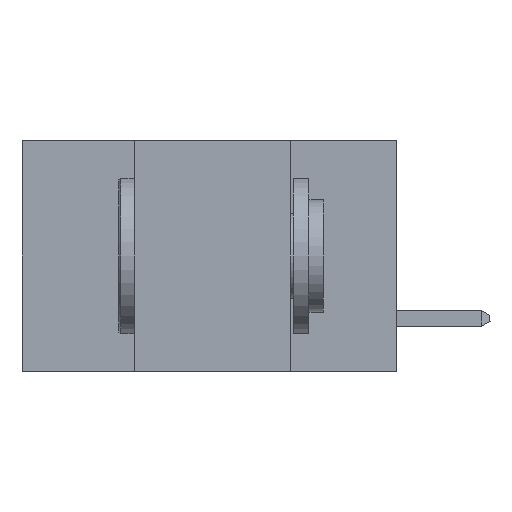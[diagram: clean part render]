
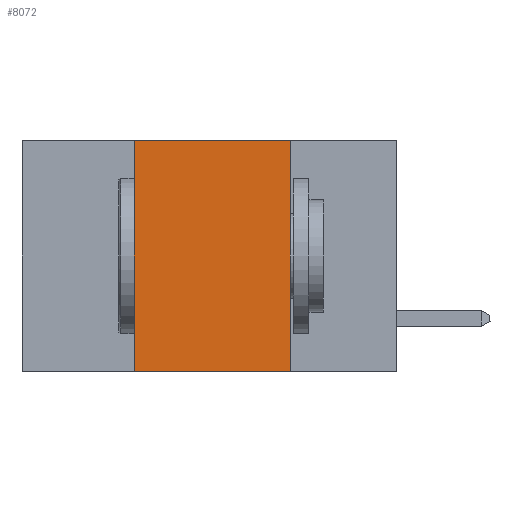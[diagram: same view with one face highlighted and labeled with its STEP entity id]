
A CAD part, left-side view. The second image highlights one B-rep face of the part: STEP entity #8072.
In plain terms, the highlighted planar face has unit normal (-1, 0, 0).
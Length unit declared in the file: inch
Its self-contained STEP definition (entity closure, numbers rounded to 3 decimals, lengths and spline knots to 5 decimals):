
#80 = ORIENTED_EDGE ( 'NONE', *, *, #22146, .F. ) ;
#754 = CARTESIAN_POINT ( 'NONE',  ( 0., 0.6, 0. ) ) ;
#1075 = CARTESIAN_POINT ( 'NONE',  ( 0., 0.42, 0. ) ) ;
#2764 = VERTEX_POINT ( 'NONE', #1075 ) ;
#4696 = ORIENTED_EDGE ( 'NONE', *, *, #19412, .F. ) ;
#4698 = PLANE ( 'NONE',  #17462 ) ;
#6309 = VECTOR ( 'NONE', #8618, 39.37008 ) ;
#6704 = CARTESIAN_POINT ( 'NONE',  ( 0., 0.42, 0. ) ) ;
#7156 = VECTOR ( 'NONE', #15991, 39.37008 ) ;
#7197 = EDGE_CURVE ( 'NONE', #15797, #23792, #11929, .T. ) ;
#8072 = ADVANCED_FACE ( 'NONE', ( #24099 ), #4698, .F. ) ;
#8540 = DIRECTION ( 'NONE',  ( 1., 0., 0. ) ) ;
#8618 = DIRECTION ( 'NONE',  ( 0., -1., 0. ) ) ;
#10206 = CARTESIAN_POINT ( 'NONE',  ( 0., 0.17, 0. ) ) ;
#11247 = ORIENTED_EDGE ( 'NONE', *, *, #17803, .F. ) ;
#11929 = LINE ( 'NONE', #21916, #6309 ) ;
#12406 = DIRECTION ( 'NONE',  ( 0., 0., -1. ) ) ;
#12696 = EDGE_LOOP ( 'NONE', ( #11247, #80, #4696, #14956 ) ) ;
#13218 = CARTESIAN_POINT ( 'NONE',  ( 0., 0.42, -0.37 ) ) ;
#13693 = LINE ( 'NONE', #6704, #13984 ) ;
#13984 = VECTOR ( 'NONE', #23913, 39.37008 ) ;
#14269 = CARTESIAN_POINT ( 'NONE',  ( 0., 0.17, 0. ) ) ;
#14956 = ORIENTED_EDGE ( 'NONE', *, *, #7197, .T. ) ;
#15109 = VERTEX_POINT ( 'NONE', #14269 ) ;
#15544 = VECTOR ( 'NONE', #21524, 39.37008 ) ;
#15797 = VERTEX_POINT ( 'NONE', #13218 ) ;
#15991 = DIRECTION ( 'NONE',  ( 0., -1., 0. ) ) ;
#16648 = CARTESIAN_POINT ( 'NONE',  ( 0., 0.17, -0.37 ) ) ;
#17462 = AXIS2_PLACEMENT_3D ( 'NONE', #19926, #8540, #12406 ) ;
#17803 = EDGE_CURVE ( 'NONE', #15109, #23792, #20602, .T. ) ;
#19412 = EDGE_CURVE ( 'NONE', #15797, #2764, #13693, .T. ) ;
#19926 = CARTESIAN_POINT ( 'NONE',  ( 0., 0.6, 0. ) ) ;
#20602 = LINE ( 'NONE', #10206, #15544 ) ;
#20839 = LINE ( 'NONE', #754, #7156 ) ;
#21524 = DIRECTION ( 'NONE',  ( 0., 0., -1. ) ) ;
#21916 = CARTESIAN_POINT ( 'NONE',  ( 0., 0.6, -0.37 ) ) ;
#22146 = EDGE_CURVE ( 'NONE', #2764, #15109, #20839, .T. ) ;
#23792 = VERTEX_POINT ( 'NONE', #16648 ) ;
#23913 = DIRECTION ( 'NONE',  ( 0., 0., 1. ) ) ;
#24099 = FACE_OUTER_BOUND ( 'NONE', #12696, .T. ) ;
